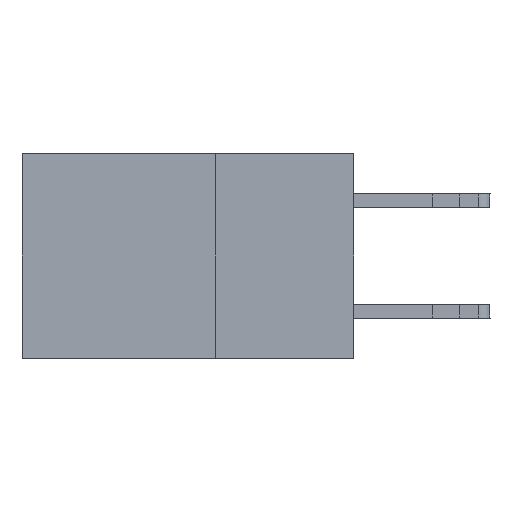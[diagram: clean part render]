
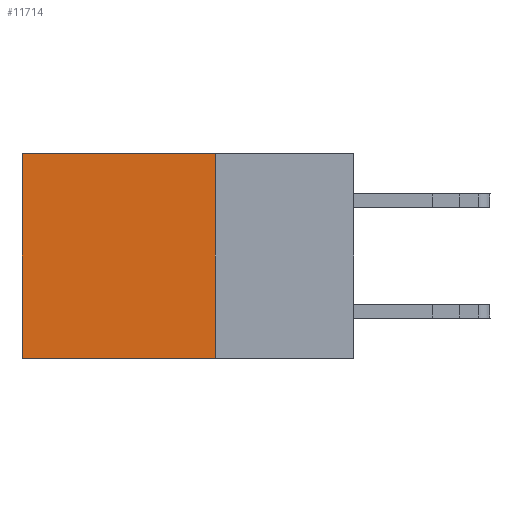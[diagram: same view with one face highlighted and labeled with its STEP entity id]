
A CAD part, left-side view. The second image highlights one B-rep face of the part: STEP entity #11714.
In plain terms, the highlighted planar face has unit normal (-1, 0, 0).
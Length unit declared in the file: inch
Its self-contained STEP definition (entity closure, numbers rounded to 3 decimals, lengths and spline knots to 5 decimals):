
#1197 = VERTEX_POINT ( 'NONE', #27206 ) ;
#2744 = ORIENTED_EDGE ( 'NONE', *, *, #21612, .T. ) ;
#3146 = LINE ( 'NONE', #24745, #15484 ) ;
#3338 = AXIS2_PLACEMENT_3D ( 'NONE', #15995, #25795, #30162 ) ;
#4321 = CARTESIAN_POINT ( 'NONE',  ( 0.2875, 0.6, -0.37 ) ) ;
#4748 = ORIENTED_EDGE ( 'NONE', *, *, #11533, .F. ) ;
#5613 = CARTESIAN_POINT ( 'NONE',  ( 0.2875, 0.25, 0. ) ) ;
#6731 = DIRECTION ( 'NONE',  ( 0., 1., 0. ) ) ;
#6989 = FACE_OUTER_BOUND ( 'NONE', #11508, .T. ) ;
#9318 = PLANE ( 'NONE',  #3338 ) ;
#11508 = EDGE_LOOP ( 'NONE', ( #2744, #30428, #4748, #23102 ) ) ;
#11533 = EDGE_CURVE ( 'NONE', #15642, #1197, #17553, .T. ) ;
#11714 = ADVANCED_FACE ( 'NONE', ( #6989 ), #9318, .F. ) ;
#12778 = VECTOR ( 'NONE', #29695, 39.37008 ) ;
#13052 = CARTESIAN_POINT ( 'NONE',  ( 0.2875, 0.6, 0. ) ) ;
#13726 = CARTESIAN_POINT ( 'NONE',  ( 0.2875, 0.25, 0. ) ) ;
#15025 = CARTESIAN_POINT ( 'NONE',  ( 0.2875, 0.6, 0. ) ) ;
#15484 = VECTOR ( 'NONE', #27234, 39.37008 ) ;
#15642 = VERTEX_POINT ( 'NONE', #19224 ) ;
#15995 = CARTESIAN_POINT ( 'NONE',  ( 0.2875, 0.25, 0. ) ) ;
#16495 = LINE ( 'NONE', #13726, #30120 ) ;
#17553 = LINE ( 'NONE', #5613, #12778 ) ;
#19224 = CARTESIAN_POINT ( 'NONE',  ( 0.2875, 0.25, 0. ) ) ;
#21612 = EDGE_CURVE ( 'NONE', #27064, #25585, #22857, .T. ) ;
#22857 = LINE ( 'NONE', #13052, #26797 ) ;
#23102 = ORIENTED_EDGE ( 'NONE', *, *, #27757, .T. ) ;
#24745 = CARTESIAN_POINT ( 'NONE',  ( 0.2875, 0.25, -0.37 ) ) ;
#24789 = EDGE_CURVE ( 'NONE', #1197, #25585, #3146, .T. ) ;
#25585 = VERTEX_POINT ( 'NONE', #4321 ) ;
#25795 = DIRECTION ( 'NONE',  ( 1., 0., 0. ) ) ;
#26797 = VECTOR ( 'NONE', #27363, 39.37008 ) ;
#27064 = VERTEX_POINT ( 'NONE', #15025 ) ;
#27206 = CARTESIAN_POINT ( 'NONE',  ( 0.2875, 0.25, -0.37 ) ) ;
#27234 = DIRECTION ( 'NONE',  ( 0., 1., 0. ) ) ;
#27363 = DIRECTION ( 'NONE',  ( 0., 0., -1. ) ) ;
#27757 = EDGE_CURVE ( 'NONE', #15642, #27064, #16495, .T. ) ;
#29695 = DIRECTION ( 'NONE',  ( 0., 0., -1. ) ) ;
#30120 = VECTOR ( 'NONE', #6731, 39.37008 ) ;
#30162 = DIRECTION ( 'NONE',  ( 0., 0., -1. ) ) ;
#30428 = ORIENTED_EDGE ( 'NONE', *, *, #24789, .F. ) ;
